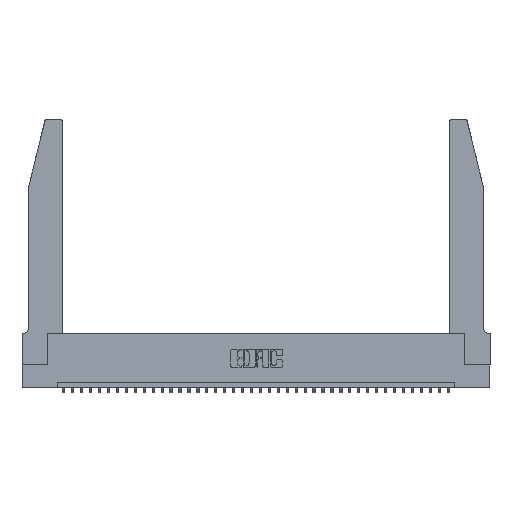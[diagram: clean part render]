
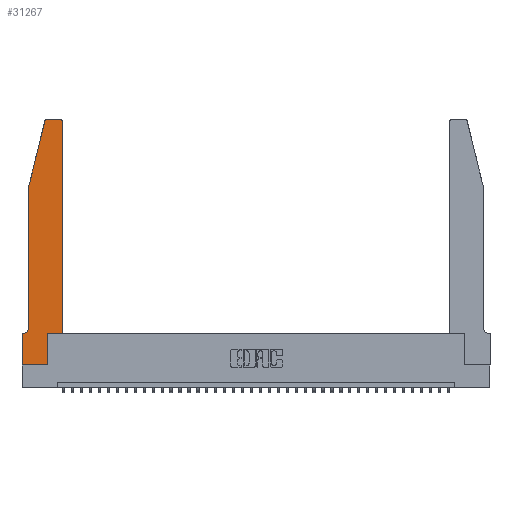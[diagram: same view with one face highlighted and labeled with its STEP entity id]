
A CAD part, top view. The second image highlights one B-rep face of the part: STEP entity #31267.
In plain terms, the highlighted planar face has unit normal (0, 0, 1).
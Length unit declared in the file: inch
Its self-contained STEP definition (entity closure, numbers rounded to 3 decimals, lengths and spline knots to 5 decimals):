
#153 = DIRECTION ( 'NONE',  ( 1., 0., 0. ) ) ;
#534 = CARTESIAN_POINT ( 'NONE',  ( 0.4205, 2.75, 0.37 ) ) ;
#1034 = DIRECTION ( 'NONE',  ( 0., 0., 1. ) ) ;
#1277 = CARTESIAN_POINT ( 'NONE',  ( 0.0755, 2., 0.37 ) ) ;
#1683 = EDGE_CURVE ( 'NONE', #9777, #27468, #15842, .T. ) ;
#1756 = ORIENTED_EDGE ( 'NONE', *, *, #15046, .T. ) ;
#1811 = VERTEX_POINT ( 'NONE', #13788 ) ;
#1841 = CARTESIAN_POINT ( 'NONE',  ( 0., 0.35, 0.37 ) ) ;
#2188 = EDGE_CURVE ( 'NONE', #29934, #22445, #24217, .T. ) ;
#2742 = LINE ( 'NONE', #9482, #31903 ) ;
#3220 = DIRECTION ( 'NONE',  ( 0., 0., 1. ) ) ;
#4089 = ORIENTED_EDGE ( 'NONE', *, *, #2188, .T. ) ;
#4424 = CARTESIAN_POINT ( 'NONE',  ( 0.25487, 2.72718, 0.37 ) ) ;
#4968 = CARTESIAN_POINT ( 'NONE',  ( 0.0755, 2., 0.37 ) ) ;
#5110 = DIRECTION ( 'NONE',  ( -0.239, -0.971, 0. ) ) ;
#5248 = CIRCLE ( 'NONE', #9120, 0.03 ) ;
#5344 = CARTESIAN_POINT ( 'NONE',  ( 0.0055, 0.35, 0.37 ) ) ;
#5738 = EDGE_CURVE ( 'NONE', #22445, #21753, #8934, .T. ) ;
#6358 = LINE ( 'NONE', #32503, #26879 ) ;
#6570 = DIRECTION ( 'NONE',  ( 1., 0., 0. ) ) ;
#6804 = ORIENTED_EDGE ( 'NONE', *, *, #14354, .T. ) ;
#7706 = ORIENTED_EDGE ( 'NONE', *, *, #8710, .T. ) ;
#8052 = CARTESIAN_POINT ( 'NONE',  ( 0.284, 2.75, 0.37 ) ) ;
#8365 = DIRECTION ( 'NONE',  ( -1., 0., 0. ) ) ;
#8710 = EDGE_CURVE ( 'NONE', #17614, #29934, #6358, .T. ) ;
#8934 = LINE ( 'NONE', #16221, #26260 ) ;
#8945 = PLANE ( 'NONE',  #23530 ) ;
#9120 = AXIS2_PLACEMENT_3D ( 'NONE', #24752, #1034, #30213 ) ;
#9482 = CARTESIAN_POINT ( 'NONE',  ( 0.4505, 0.35, 0.37 ) ) ;
#9777 = VERTEX_POINT ( 'NONE', #5344 ) ;
#10164 = DIRECTION ( 'NONE',  ( -1., 0., 0. ) ) ;
#11058 = LINE ( 'NONE', #21153, #17363 ) ;
#11695 = LINE ( 'NONE', #1277, #29420 ) ;
#12631 = LINE ( 'NONE', #29370, #24001 ) ;
#13671 = ORIENTED_EDGE ( 'NONE', *, *, #37188, .T. ) ;
#13788 = CARTESIAN_POINT ( 'NONE',  ( 0.0755, 0.42, 0.37 ) ) ;
#13977 = CARTESIAN_POINT ( 'NONE',  ( 0.0055, 0.42, 0.37 ) ) ;
#14354 = EDGE_CURVE ( 'NONE', #35151, #36182, #2742, .T. ) ;
#15046 = EDGE_CURVE ( 'NONE', #32805, #35151, #12631, .T. ) ;
#15788 = ORIENTED_EDGE ( 'NONE', *, *, #27899, .T. ) ;
#15842 = LINE ( 'NONE', #20322, #35325 ) ;
#16221 = CARTESIAN_POINT ( 'NONE',  ( 0.0755, 2., 0.37 ) ) ;
#16717 = VECTOR ( 'NONE', #37191, 39.37008 ) ;
#17018 = ORIENTED_EDGE ( 'NONE', *, *, #1683, .T. ) ;
#17363 = VECTOR ( 'NONE', #23665, 39.37008 ) ;
#17614 = VERTEX_POINT ( 'NONE', #534 ) ;
#18354 = DIRECTION ( 'NONE',  ( 1., 0., 0. ) ) ;
#19675 = CIRCLE ( 'NONE', #31983, 0.07 ) ;
#20322 = CARTESIAN_POINT ( 'NONE',  ( 0.0755, 0.35, 0.37 ) ) ;
#20579 = CARTESIAN_POINT ( 'NONE',  ( 0., 0.35, 0.37 ) ) ;
#20750 = FACE_OUTER_BOUND ( 'NONE', #29315, .T. ) ;
#21047 = VECTOR ( 'NONE', #30407, 39.37008 ) ;
#21153 = CARTESIAN_POINT ( 'NONE',  ( 0., 0., 0.37 ) ) ;
#21753 = VERTEX_POINT ( 'NONE', #4968 ) ;
#21953 = ORIENTED_EDGE ( 'NONE', *, *, #23825, .T. ) ;
#22445 = VERTEX_POINT ( 'NONE', #4424 ) ;
#22730 = CARTESIAN_POINT ( 'NONE',  ( 0.4505, 2.72, 0.37 ) ) ;
#22864 = ORIENTED_EDGE ( 'NONE', *, *, #5738, .T. ) ;
#23530 = AXIS2_PLACEMENT_3D ( 'NONE', #20579, #3220, #153 ) ;
#23665 = DIRECTION ( 'NONE',  ( 0., -1., 0. ) ) ;
#23825 = EDGE_CURVE ( 'NONE', #36182, #17614, #5248, .T. ) ;
#23952 = ORIENTED_EDGE ( 'NONE', *, *, #30991, .T. ) ;
#24001 = VECTOR ( 'NONE', #6570, 39.37008 ) ;
#24217 = CIRCLE ( 'NONE', #26405, 0.03 ) ;
#24752 = CARTESIAN_POINT ( 'NONE',  ( 0.4205, 2.72, 0.37 ) ) ;
#25548 = CARTESIAN_POINT ( 'NONE',  ( 0.2865, 0.35, 0.37 ) ) ;
#25591 = CARTESIAN_POINT ( 'NONE',  ( 0.4505, 0.35, 0.37 ) ) ;
#26260 = VECTOR ( 'NONE', #5110, 39.37008 ) ;
#26405 = AXIS2_PLACEMENT_3D ( 'NONE', #30196, #29933, #18354 ) ;
#26677 = EDGE_CURVE ( 'NONE', #34282, #31683, #28795, .T. ) ;
#26879 = VECTOR ( 'NONE', #35519, 39.37008 ) ;
#27089 = CARTESIAN_POINT ( 'NONE',  ( 0., 0., 0.37 ) ) ;
#27289 = ORIENTED_EDGE ( 'NONE', *, *, #26677, .T. ) ;
#27376 = DIRECTION ( 'NONE',  ( 0., -1., 0. ) ) ;
#27468 = VERTEX_POINT ( 'NONE', #1841 ) ;
#27738 = DIRECTION ( 'NONE',  ( 0., 1., 0. ) ) ;
#27899 = EDGE_CURVE ( 'NONE', #27468, #34282, #11058, .T. ) ;
#28001 = ORIENTED_EDGE ( 'NONE', *, *, #28776, .T. ) ;
#28776 = EDGE_CURVE ( 'NONE', #1811, #9777, #19675, .T. ) ;
#28795 = LINE ( 'NONE', #27089, #21047 ) ;
#28922 = CARTESIAN_POINT ( 'NONE',  ( 0.2865, 0.35, 0.37 ) ) ;
#29315 = EDGE_LOOP ( 'NONE', ( #7706, #4089, #22864, #13671, #28001, #17018, #15788, #27289, #23952, #1756, #6804, #21953 ) ) ;
#29370 = CARTESIAN_POINT ( 'NONE',  ( 0.4505, 0.35, 0.37 ) ) ;
#29420 = VECTOR ( 'NONE', #27376, 39.37008 ) ;
#29933 = DIRECTION ( 'NONE',  ( 0., 0., 1. ) ) ;
#29934 = VERTEX_POINT ( 'NONE', #8052 ) ;
#30196 = CARTESIAN_POINT ( 'NONE',  ( 0.284, 2.72, 0.37 ) ) ;
#30213 = DIRECTION ( 'NONE',  ( 1., 0., 0. ) ) ;
#30359 = CARTESIAN_POINT ( 'NONE',  ( 0., 0., 0.37 ) ) ;
#30407 = DIRECTION ( 'NONE',  ( 1., 0., 0. ) ) ;
#30991 = EDGE_CURVE ( 'NONE', #31683, #32805, #33545, .T. ) ;
#31267 = ADVANCED_FACE ( 'NONE', ( #20750 ), #8945, .T. ) ;
#31668 = DIRECTION ( 'NONE',  ( 0., 0., -1. ) ) ;
#31683 = VERTEX_POINT ( 'NONE', #36546 ) ;
#31903 = VECTOR ( 'NONE', #27738, 39.37008 ) ;
#31983 = AXIS2_PLACEMENT_3D ( 'NONE', #13977, #31668, #8365 ) ;
#32503 = CARTESIAN_POINT ( 'NONE',  ( 0.2605, 2.75, 0.37 ) ) ;
#32805 = VERTEX_POINT ( 'NONE', #28922 ) ;
#33545 = LINE ( 'NONE', #25548, #16717 ) ;
#34282 = VERTEX_POINT ( 'NONE', #30359 ) ;
#35151 = VERTEX_POINT ( 'NONE', #25591 ) ;
#35325 = VECTOR ( 'NONE', #10164, 39.37008 ) ;
#35519 = DIRECTION ( 'NONE',  ( -1., 0., 0. ) ) ;
#36182 = VERTEX_POINT ( 'NONE', #22730 ) ;
#36546 = CARTESIAN_POINT ( 'NONE',  ( 0.2865, 0., 0.37 ) ) ;
#37188 = EDGE_CURVE ( 'NONE', #21753, #1811, #11695, .T. ) ;
#37191 = DIRECTION ( 'NONE',  ( 0., 1., 0. ) ) ;
